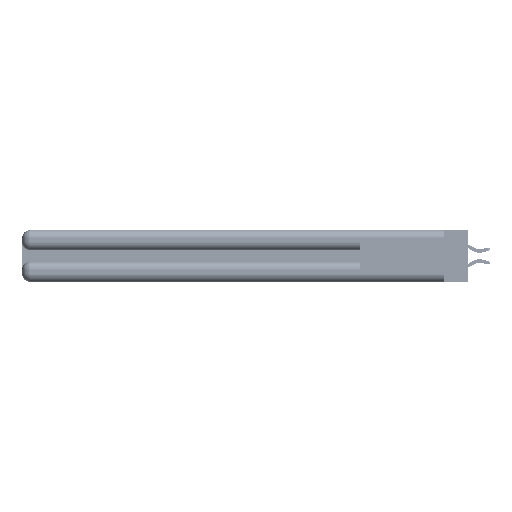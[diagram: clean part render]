
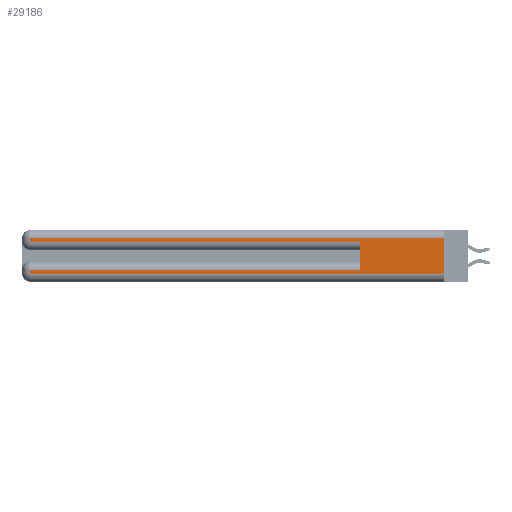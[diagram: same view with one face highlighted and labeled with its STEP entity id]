
A CAD part, left-side view. The second image highlights one B-rep face of the part: STEP entity #29186.
In plain terms, the highlighted planar face has unit normal (-1, 0, 0).
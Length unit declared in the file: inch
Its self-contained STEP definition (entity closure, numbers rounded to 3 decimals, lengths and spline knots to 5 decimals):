
#1037 = LINE ( 'NONE', #51526, #34416 ) ;
#2116 = EDGE_CURVE ( 'NONE', #33381, #27240, #1037, .T. ) ;
#2359 = FACE_OUTER_BOUND ( 'NONE', #31545, .T. ) ;
#4041 = CARTESIAN_POINT ( 'NONE',  ( 0., 0., 0.285 ) ) ;
#4215 = VECTOR ( 'NONE', #17898, 39.37008 ) ;
#4469 = LINE ( 'NONE', #9183, #25434 ) ;
#4611 = LINE ( 'NONE', #4041, #46521 ) ;
#7277 = VERTEX_POINT ( 'NONE', #15621 ) ;
#7803 = CARTESIAN_POINT ( 'NONE',  ( 0., 0., 0.31 ) ) ;
#7809 = ORIENTED_EDGE ( 'NONE', *, *, #52638, .T. ) ;
#8657 = VERTEX_POINT ( 'NONE', #7803 ) ;
#9183 = CARTESIAN_POINT ( 'NONE',  ( 0., 0., 0.06 ) ) ;
#9882 = VECTOR ( 'NONE', #21404, 39.37008 ) ;
#9908 = LINE ( 'NONE', #21439, #42011 ) ;
#13415 = DIRECTION ( 'NONE',  ( 0., -1., 0. ) ) ;
#15020 = DIRECTION ( 'NONE',  ( 0., 0., -1. ) ) ;
#15330 = CARTESIAN_POINT ( 'NONE',  ( 0., 0.6, 0.085 ) ) ;
#15621 = CARTESIAN_POINT ( 'NONE',  ( 0., 0., 0.06 ) ) ;
#16495 = EDGE_CURVE ( 'NONE', #8657, #49919, #9908, .T. ) ;
#17781 = EDGE_CURVE ( 'NONE', #28937, #27240, #4611, .T. ) ;
#17898 = DIRECTION ( 'NONE',  ( 0., 1., 0. ) ) ;
#18436 = DIRECTION ( 'NONE',  ( 1., 0., 0. ) ) ;
#19641 = CARTESIAN_POINT ( 'NONE',  ( 0., 2.94, 0.37 ) ) ;
#21041 = LINE ( 'NONE', #38065, #9882 ) ;
#21160 = CARTESIAN_POINT ( 'NONE',  ( 0., 2.94, 0.06 ) ) ;
#21404 = DIRECTION ( 'NONE',  ( 0., 0., -1. ) ) ;
#21439 = CARTESIAN_POINT ( 'NONE',  ( 0., 0., 0.31 ) ) ;
#22242 = AXIS2_PLACEMENT_3D ( 'NONE', #22455, #18436, #47665 ) ;
#22455 = CARTESIAN_POINT ( 'NONE',  ( 0., 0., 0.37 ) ) ;
#22485 = VERTEX_POINT ( 'NONE', #21160 ) ;
#22896 = CARTESIAN_POINT ( 'NONE',  ( 0., 2.94, 0.285 ) ) ;
#23654 = VECTOR ( 'NONE', #44867, 39.37008 ) ;
#24174 = ORIENTED_EDGE ( 'NONE', *, *, #28996, .F. ) ;
#25434 = VECTOR ( 'NONE', #13415, 39.37008 ) ;
#26444 = ORIENTED_EDGE ( 'NONE', *, *, #2116, .F. ) ;
#27240 = VERTEX_POINT ( 'NONE', #36938 ) ;
#28937 = VERTEX_POINT ( 'NONE', #22896 ) ;
#28996 = EDGE_CURVE ( 'NONE', #8657, #7277, #53386, .T. ) ;
#29132 = LINE ( 'NONE', #34547, #4215 ) ;
#29186 = ADVANCED_FACE ( 'NONE', ( #2359 ), #43490, .F. ) ;
#29473 = ORIENTED_EDGE ( 'NONE', *, *, #46751, .T. ) ;
#31545 = EDGE_LOOP ( 'NONE', ( #24174, #45672, #7809, #44446, #26444, #29473, #39837, #38254 ) ) ;
#33381 = VERTEX_POINT ( 'NONE', #15330 ) ;
#34416 = VECTOR ( 'NONE', #43356, 39.37008 ) ;
#34547 = CARTESIAN_POINT ( 'NONE',  ( 0., 0., 0.085 ) ) ;
#34798 = LINE ( 'NONE', #19641, #23654 ) ;
#36938 = CARTESIAN_POINT ( 'NONE',  ( 0., 0.6, 0.285 ) ) ;
#38065 = CARTESIAN_POINT ( 'NONE',  ( 0., 2.94, 0.37 ) ) ;
#38254 = ORIENTED_EDGE ( 'NONE', *, *, #43703, .T. ) ;
#38902 = VERTEX_POINT ( 'NONE', #53274 ) ;
#39572 = EDGE_CURVE ( 'NONE', #38902, #22485, #34798, .T. ) ;
#39837 = ORIENTED_EDGE ( 'NONE', *, *, #39572, .T. ) ;
#41792 = CARTESIAN_POINT ( 'NONE',  ( 0., 2.94, 0.31 ) ) ;
#42011 = VECTOR ( 'NONE', #50830, 39.37008 ) ;
#42324 = VECTOR ( 'NONE', #15020, 39.37008 ) ;
#43356 = DIRECTION ( 'NONE',  ( 0., 0., 1. ) ) ;
#43490 = PLANE ( 'NONE',  #22242 ) ;
#43703 = EDGE_CURVE ( 'NONE', #22485, #7277, #4469, .T. ) ;
#44446 = ORIENTED_EDGE ( 'NONE', *, *, #17781, .T. ) ;
#44867 = DIRECTION ( 'NONE',  ( 0., 0., -1. ) ) ;
#45672 = ORIENTED_EDGE ( 'NONE', *, *, #16495, .T. ) ;
#45780 = DIRECTION ( 'NONE',  ( 0., -1., 0. ) ) ;
#46521 = VECTOR ( 'NONE', #45780, 39.37008 ) ;
#46751 = EDGE_CURVE ( 'NONE', #33381, #38902, #29132, .T. ) ;
#47665 = DIRECTION ( 'NONE',  ( 0., 0., -1. ) ) ;
#48466 = CARTESIAN_POINT ( 'NONE',  ( 0., 0., 0.37 ) ) ;
#49919 = VERTEX_POINT ( 'NONE', #41792 ) ;
#50830 = DIRECTION ( 'NONE',  ( 0., 1., 0. ) ) ;
#51526 = CARTESIAN_POINT ( 'NONE',  ( 0., 0.6, 0.145 ) ) ;
#52638 = EDGE_CURVE ( 'NONE', #49919, #28937, #21041, .T. ) ;
#53274 = CARTESIAN_POINT ( 'NONE',  ( 0., 2.94, 0.085 ) ) ;
#53386 = LINE ( 'NONE', #48466, #42324 ) ;
